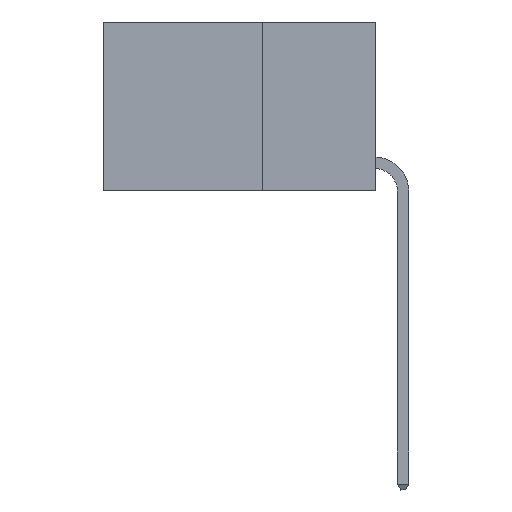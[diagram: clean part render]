
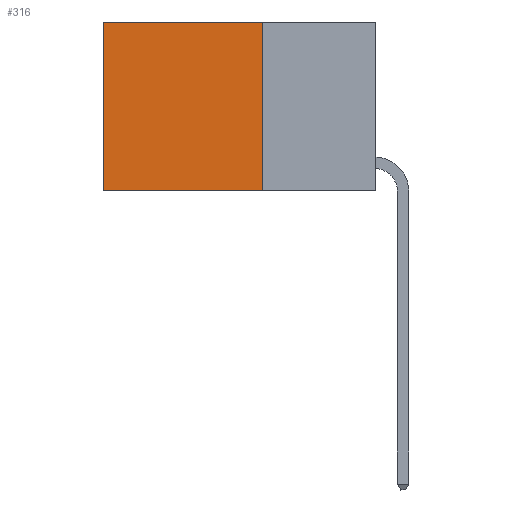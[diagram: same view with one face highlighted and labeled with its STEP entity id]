
A CAD part, left-side view. The second image highlights one B-rep face of the part: STEP entity #316.
In plain terms, the highlighted planar face has unit normal (-1, 0, 0).
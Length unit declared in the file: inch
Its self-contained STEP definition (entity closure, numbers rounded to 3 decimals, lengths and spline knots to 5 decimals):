
#316 = ADVANCED_FACE ( 'NONE', ( #1890 ), #1058, .F. ) ;
#538 = LINE ( 'NONE', #7377, #811 ) ;
#681 = DIRECTION ( 'NONE',  ( 0., 1., 0. ) ) ;
#811 = VECTOR ( 'NONE', #10750, 39.37008 ) ;
#907 = LINE ( 'NONE', #10084, #8058 ) ;
#1058 = PLANE ( 'NONE',  #10397 ) ;
#1310 = CARTESIAN_POINT ( 'NONE',  ( 0.2625, 0.25, -0.37 ) ) ;
#1890 = FACE_OUTER_BOUND ( 'NONE', #4513, .T. ) ;
#1978 = ORIENTED_EDGE ( 'NONE', *, *, #6578, .F. ) ;
#2686 = CARTESIAN_POINT ( 'NONE',  ( 0.2625, 0.6, 0. ) ) ;
#2867 = VERTEX_POINT ( 'NONE', #10643 ) ;
#2888 = VECTOR ( 'NONE', #4693, 39.37008 ) ;
#3485 = ORIENTED_EDGE ( 'NONE', *, *, #7340, .T. ) ;
#4045 = CARTESIAN_POINT ( 'NONE',  ( 0.2625, 0.25, 0. ) ) ;
#4513 = EDGE_LOOP ( 'NONE', ( #3485, #8994, #1978, #11018 ) ) ;
#4693 = DIRECTION ( 'NONE',  ( 0., 1., 0. ) ) ;
#4762 = VECTOR ( 'NONE', #8706, 39.37008 ) ;
#5073 = EDGE_CURVE ( 'NONE', #9808, #2867, #5552, .T. ) ;
#5528 = VERTEX_POINT ( 'NONE', #4045 ) ;
#5552 = LINE ( 'NONE', #1310, #2888 ) ;
#5817 = EDGE_CURVE ( 'NONE', #5528, #7662, #907, .T. ) ;
#6029 = CARTESIAN_POINT ( 'NONE',  ( 0.2625, 0.25, 0. ) ) ;
#6578 = EDGE_CURVE ( 'NONE', #5528, #9808, #538, .T. ) ;
#6847 = CARTESIAN_POINT ( 'NONE',  ( 0.2625, 0.25, -0.37 ) ) ;
#7340 = EDGE_CURVE ( 'NONE', #7662, #2867, #10405, .T. ) ;
#7377 = CARTESIAN_POINT ( 'NONE',  ( 0.2625, 0.25, 0. ) ) ;
#7662 = VERTEX_POINT ( 'NONE', #7677 ) ;
#7677 = CARTESIAN_POINT ( 'NONE',  ( 0.2625, 0.6, 0. ) ) ;
#7953 = DIRECTION ( 'NONE',  ( 1., 0., 0. ) ) ;
#8058 = VECTOR ( 'NONE', #681, 39.37008 ) ;
#8706 = DIRECTION ( 'NONE',  ( 0., 0., -1. ) ) ;
#8740 = DIRECTION ( 'NONE',  ( 0., 0., -1. ) ) ;
#8994 = ORIENTED_EDGE ( 'NONE', *, *, #5073, .F. ) ;
#9808 = VERTEX_POINT ( 'NONE', #6847 ) ;
#10084 = CARTESIAN_POINT ( 'NONE',  ( 0.2625, 0.25, 0. ) ) ;
#10397 = AXIS2_PLACEMENT_3D ( 'NONE', #6029, #7953, #8740 ) ;
#10405 = LINE ( 'NONE', #2686, #4762 ) ;
#10643 = CARTESIAN_POINT ( 'NONE',  ( 0.2625, 0.6, -0.37 ) ) ;
#10750 = DIRECTION ( 'NONE',  ( 0., 0., -1. ) ) ;
#11018 = ORIENTED_EDGE ( 'NONE', *, *, #5817, .T. ) ;
